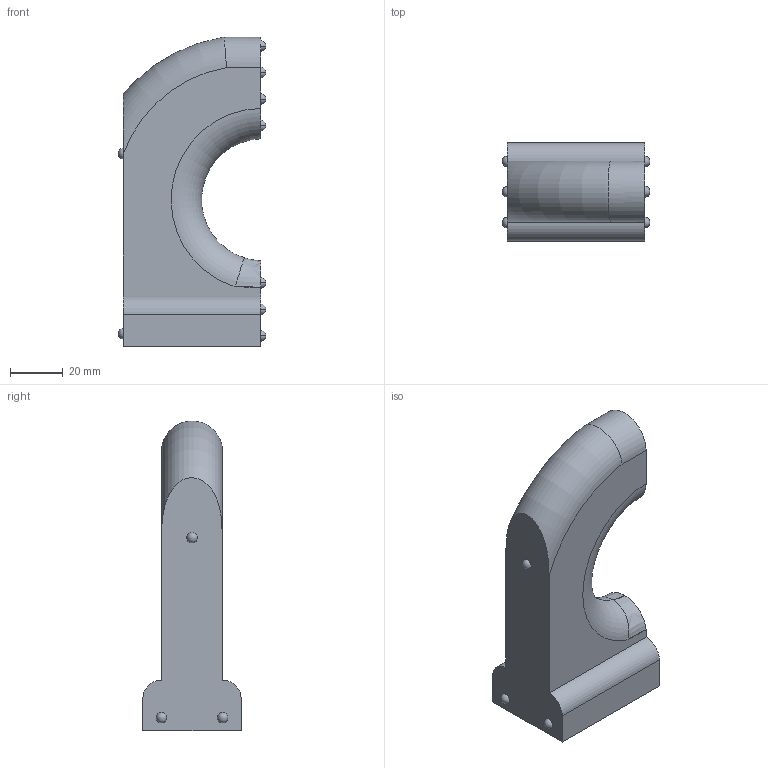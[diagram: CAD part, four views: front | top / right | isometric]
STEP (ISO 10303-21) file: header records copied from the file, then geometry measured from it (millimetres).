
FILE_DESCRIPTION (( 'STEP AP214' ), '1' );
FILE_NAME ('Charon_V3_Pistol_1.STEP', '2013-09-01T16:55:53', ( 'Asher' ), ( '' ), 'SwSTEP 2.0', 'SolidWorks 2013', '' );
FILE_SCHEMA (( 'AUTOMOTIVE_DESIGN' ));
Length unit declared in the file: millimetre
Products named in the file (1): Charon_V3_Pistol_1
Bounding box: 55.83 x 37.13 x 117.02 mm (x, y, z)
Volume: 119700.8 mm3; surface area: 18420.3 mm2
Topology: 1 solids, 1 shells, 55 faces, 186 edges, 119 vertices
Faces by surface type: sphere 34, plane 8, bspline 6, cylinder 4, torus 3
Entity records: 1903 total; most frequent: CARTESIAN_POINT 665, DIRECTION 266, ORIENTED_EDGE 224, AXIS2_PLACEMENT_3D 122, EDGE_CURVE 112, VERTEX_POINT 82, EDGE_LOOP 78, CIRCLE 72
